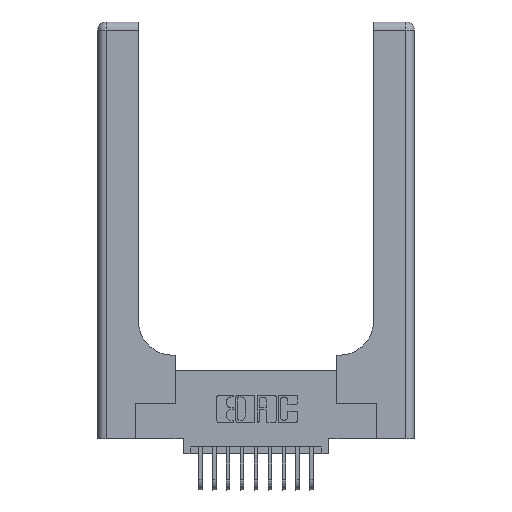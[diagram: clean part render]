
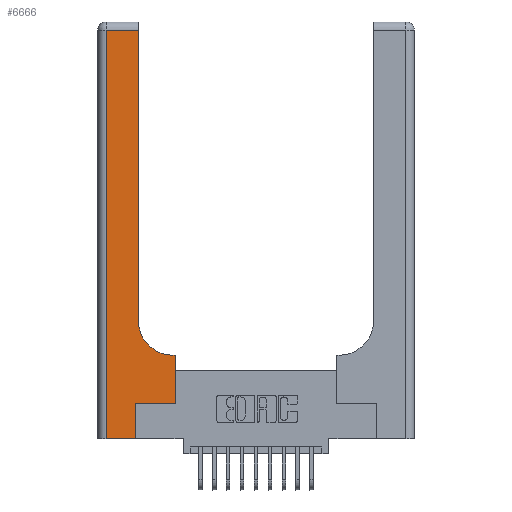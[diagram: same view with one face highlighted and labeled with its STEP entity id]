
A CAD part, top view. The second image highlights one B-rep face of the part: STEP entity #6666.
In plain terms, the highlighted planar face has unit normal (0, 0, 1).
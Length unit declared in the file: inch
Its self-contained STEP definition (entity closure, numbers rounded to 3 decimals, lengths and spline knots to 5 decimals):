
#43 = CARTESIAN_POINT ( 'NONE',  ( 0.5585, 0.6, 0.37 ) ) ;
#391 = CARTESIAN_POINT ( 'NONE',  ( 0.2915, 2.94, 0.37 ) ) ;
#661 = CARTESIAN_POINT ( 'NONE',  ( 0.06, 3., 0.37 ) ) ;
#801 = DIRECTION ( 'NONE',  ( 0., 1., 0. ) ) ;
#853 = CARTESIAN_POINT ( 'NONE',  ( 0.06, 0., 0.37 ) ) ;
#894 = CARTESIAN_POINT ( 'NONE',  ( 0.2915, 0.6, 0.37 ) ) ;
#1176 = VECTOR ( 'NONE', #11708, 39.37008 ) ;
#1380 = CARTESIAN_POINT ( 'NONE',  ( 0.06, 2.94, 0.37 ) ) ;
#1564 = VECTOR ( 'NONE', #10729, 39.37008 ) ;
#1839 = CARTESIAN_POINT ( 'NONE',  ( 0.269, 0.25, 0.37 ) ) ;
#1942 = DIRECTION ( 'NONE',  ( -1., 0., 0. ) ) ;
#2233 = LINE ( 'NONE', #10912, #1564 ) ;
#2284 = LINE ( 'NONE', #1839, #1176 ) ;
#2431 = VERTEX_POINT ( 'NONE', #6481 ) ;
#2446 = CARTESIAN_POINT ( 'NONE',  ( 0.269, 0.25, 0.37 ) ) ;
#2522 = DIRECTION ( 'NONE',  ( 0., 1., 0. ) ) ;
#2680 = VERTEX_POINT ( 'NONE', #2446 ) ;
#3486 = EDGE_CURVE ( 'NONE', #11046, #9386, #2233, .T. ) ;
#3787 = AXIS2_PLACEMENT_3D ( 'NONE', #11755, #14704, #7593 ) ;
#4457 = ORIENTED_EDGE ( 'NONE', *, *, #11982, .T. ) ;
#4726 = CARTESIAN_POINT ( 'NONE',  ( 0.5585, 0.25, 0.37 ) ) ;
#5572 = LINE ( 'NONE', #661, #14228 ) ;
#6191 = CARTESIAN_POINT ( 'NONE',  ( 0., 0., 0.37 ) ) ;
#6481 = CARTESIAN_POINT ( 'NONE',  ( 0.5415, 0.6, 0.37 ) ) ;
#6666 = ADVANCED_FACE ( 'NONE', ( #7756 ), #14586, .F. ) ;
#6741 = EDGE_CURVE ( 'NONE', #16390, #2680, #16424, .T. ) ;
#6758 = DIRECTION ( 'NONE',  ( 0., 0., -1. ) ) ;
#7414 = VECTOR ( 'NONE', #15182, 39.37008 ) ;
#7593 = DIRECTION ( 'NONE',  ( -1., 0., 0. ) ) ;
#7653 = CARTESIAN_POINT ( 'NONE',  ( 0., 2.94, 0.37 ) ) ;
#7756 = FACE_OUTER_BOUND ( 'NONE', #14388, .T. ) ;
#7764 = CARTESIAN_POINT ( 'NONE',  ( 0.269, 0., 0.37 ) ) ;
#7977 = CARTESIAN_POINT ( 'NONE',  ( 0.269, 0., 0.37 ) ) ;
#8899 = ORIENTED_EDGE ( 'NONE', *, *, #13698, .T. ) ;
#9267 = ORIENTED_EDGE ( 'NONE', *, *, #16508, .T. ) ;
#9289 = ORIENTED_EDGE ( 'NONE', *, *, #13312, .T. ) ;
#9373 = LINE ( 'NONE', #6191, #11797 ) ;
#9386 = VERTEX_POINT ( 'NONE', #391 ) ;
#9420 = LINE ( 'NONE', #894, #7414 ) ;
#9502 = CIRCLE ( 'NONE', #13005, 0.25 ) ;
#10000 = ORIENTED_EDGE ( 'NONE', *, *, #17202, .T. ) ;
#10729 = DIRECTION ( 'NONE',  ( 0., 1., 0. ) ) ;
#10912 = CARTESIAN_POINT ( 'NONE',  ( 0.2915, 3., 0.37 ) ) ;
#10942 = EDGE_CURVE ( 'NONE', #13350, #2431, #9420, .T. ) ;
#11035 = CARTESIAN_POINT ( 'NONE',  ( 0.5585, 0.25, 0.37 ) ) ;
#11046 = VERTEX_POINT ( 'NONE', #14414 ) ;
#11343 = VECTOR ( 'NONE', #1942, 39.37008 ) ;
#11708 = DIRECTION ( 'NONE',  ( 1., 0., 0. ) ) ;
#11755 = CARTESIAN_POINT ( 'NONE',  ( 0., 3., 0.37 ) ) ;
#11797 = VECTOR ( 'NONE', #11864, 39.37008 ) ;
#11864 = DIRECTION ( 'NONE',  ( 1., 0., 0. ) ) ;
#11945 = VECTOR ( 'NONE', #2522, 39.37008 ) ;
#11977 = VECTOR ( 'NONE', #801, 39.37008 ) ;
#11982 = EDGE_CURVE ( 'NONE', #17940, #12059, #5572, .T. ) ;
#12059 = VERTEX_POINT ( 'NONE', #853 ) ;
#12426 = LINE ( 'NONE', #7653, #11343 ) ;
#12498 = ORIENTED_EDGE ( 'NONE', *, *, #18421, .T. ) ;
#12678 = VERTEX_POINT ( 'NONE', #4726 ) ;
#13005 = AXIS2_PLACEMENT_3D ( 'NONE', #13863, #6758, #13681 ) ;
#13312 = EDGE_CURVE ( 'NONE', #9386, #17940, #12426, .T. ) ;
#13350 = VERTEX_POINT ( 'NONE', #43 ) ;
#13634 = DIRECTION ( 'NONE',  ( 0., -1., 0. ) ) ;
#13681 = DIRECTION ( 'NONE',  ( 1., 0., 0. ) ) ;
#13698 = EDGE_CURVE ( 'NONE', #12059, #16390, #9373, .T. ) ;
#13863 = CARTESIAN_POINT ( 'NONE',  ( 0.5415, 0.85, 0.37 ) ) ;
#14228 = VECTOR ( 'NONE', #13634, 39.37008 ) ;
#14388 = EDGE_LOOP ( 'NONE', ( #15208, #9289, #4457, #8899, #15662, #12498, #10000, #15862, #9267 ) ) ;
#14414 = CARTESIAN_POINT ( 'NONE',  ( 0.2915, 0.85, 0.37 ) ) ;
#14586 = PLANE ( 'NONE',  #3787 ) ;
#14704 = DIRECTION ( 'NONE',  ( 0., 0., -1. ) ) ;
#15182 = DIRECTION ( 'NONE',  ( -1., 0., 0. ) ) ;
#15208 = ORIENTED_EDGE ( 'NONE', *, *, #3486, .T. ) ;
#15258 = LINE ( 'NONE', #11035, #11945 ) ;
#15662 = ORIENTED_EDGE ( 'NONE', *, *, #6741, .T. ) ;
#15862 = ORIENTED_EDGE ( 'NONE', *, *, #10942, .T. ) ;
#16390 = VERTEX_POINT ( 'NONE', #7764 ) ;
#16424 = LINE ( 'NONE', #7977, #11977 ) ;
#16508 = EDGE_CURVE ( 'NONE', #2431, #11046, #9502, .T. ) ;
#17202 = EDGE_CURVE ( 'NONE', #12678, #13350, #15258, .T. ) ;
#17940 = VERTEX_POINT ( 'NONE', #1380 ) ;
#18421 = EDGE_CURVE ( 'NONE', #2680, #12678, #2284, .T. ) ;
